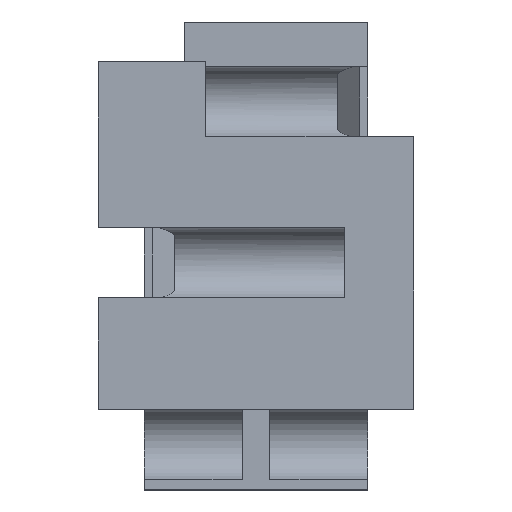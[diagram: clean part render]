
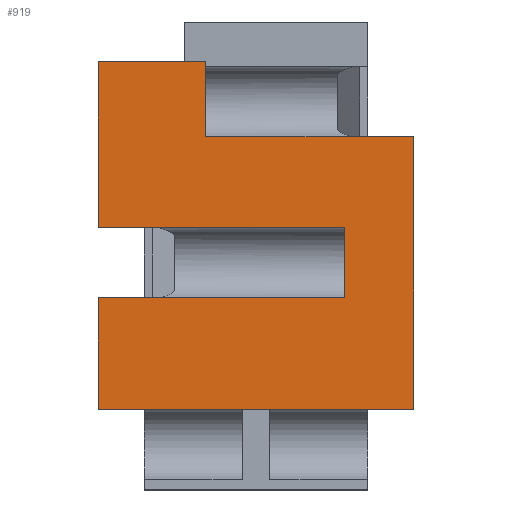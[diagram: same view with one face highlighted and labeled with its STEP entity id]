
A CAD part, top view. The second image highlights one B-rep face of the part: STEP entity #919.
In plain terms, the highlighted planar face has unit normal (0, 0, 1).
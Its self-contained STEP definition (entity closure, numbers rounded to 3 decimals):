
#56=FACE_OUTER_BOUND('',#102,.T.);
#102=EDGE_LOOP('',(#657,#658,#659,#660,#661,#662,#663,#664,#665,#666));
#169=LINE('',#1359,#286);
#174=LINE('',#1369,#291);
#177=LINE('',#1375,#294);
#181=LINE('',#1383,#298);
#183=LINE('',#1387,#300);
#184=LINE('',#1389,#301);
#185=LINE('',#1390,#302);
#186=LINE('',#1391,#303);
#187=LINE('',#1393,#304);
#188=LINE('',#1394,#305);
#286=VECTOR('',#1093,10.);
#291=VECTOR('',#1100,10.);
#294=VECTOR('',#1105,10.);
#298=VECTOR('',#1111,10.);
#300=VECTOR('',#1115,10.);
#301=VECTOR('',#1116,10.);
#302=VECTOR('',#1117,10.);
#303=VECTOR('',#1118,10.);
#304=VECTOR('',#1119,10.);
#305=VECTOR('',#1120,10.);
#400=VERTEX_POINT('',#1356);
#401=VERTEX_POINT('',#1358);
#404=VERTEX_POINT('',#1366);
#405=VERTEX_POINT('',#1368);
#406=VERTEX_POINT('',#1372);
#407=VERTEX_POINT('',#1374);
#410=VERTEX_POINT('',#1382);
#411=VERTEX_POINT('',#1386);
#412=VERTEX_POINT('',#1388);
#413=VERTEX_POINT('',#1392);
#495=EDGE_CURVE('',#401,#400,#169,.T.);
#500=EDGE_CURVE('',#405,#404,#174,.T.);
#503=EDGE_CURVE('',#407,#406,#177,.T.);
#507=EDGE_CURVE('',#410,#407,#181,.T.);
#509=EDGE_CURVE('',#406,#411,#183,.T.);
#510=EDGE_CURVE('',#411,#412,#184,.T.);
#511=EDGE_CURVE('',#412,#405,#185,.T.);
#512=EDGE_CURVE('',#404,#401,#186,.T.);
#513=EDGE_CURVE('',#400,#413,#187,.T.);
#514=EDGE_CURVE('',#413,#410,#188,.T.);
#657=ORIENTED_EDGE('',*,*,#507,.T.);
#658=ORIENTED_EDGE('',*,*,#503,.T.);
#659=ORIENTED_EDGE('',*,*,#509,.T.);
#660=ORIENTED_EDGE('',*,*,#510,.T.);
#661=ORIENTED_EDGE('',*,*,#511,.T.);
#662=ORIENTED_EDGE('',*,*,#500,.T.);
#663=ORIENTED_EDGE('',*,*,#512,.T.);
#664=ORIENTED_EDGE('',*,*,#495,.T.);
#665=ORIENTED_EDGE('',*,*,#513,.T.);
#666=ORIENTED_EDGE('',*,*,#514,.T.);
#876=PLANE('',#982);
#919=ADVANCED_FACE('',(#56),#876,.T.);
#982=AXIS2_PLACEMENT_3D('',#1385,#1113,#1114);
#1093=DIRECTION('',(0.,1.,0.));
#1100=DIRECTION('',(0.,-1.,0.));
#1105=DIRECTION('',(0.,-1.,0.));
#1111=DIRECTION('',(-1.,0.,0.));
#1113=DIRECTION('center_axis',(0.,0.,1.));
#1114=DIRECTION('ref_axis',(1.,0.,0.));
#1115=DIRECTION('',(1.,0.,0.));
#1116=DIRECTION('',(0.,-1.,0.));
#1117=DIRECTION('',(-1.,0.,0.));
#1118=DIRECTION('',(1.,0.,0.));
#1119=DIRECTION('',(-1.,0.,0.));
#1120=DIRECTION('',(0.,1.,0.));
#1356=CARTESIAN_POINT('',(10.3,9.072,11.));
#1358=CARTESIAN_POINT('',(10.3,-8.72,11.));
#1359=CARTESIAN_POINT('',(10.3,9.072,11.));
#1366=CARTESIAN_POINT('',(-10.3,-8.72,11.));
#1368=CARTESIAN_POINT('',(-10.3,-1.458,11.));
#1369=CARTESIAN_POINT('',(-10.3,-1.458,11.));
#1372=CARTESIAN_POINT('',(-10.3,3.142,11.));
#1374=CARTESIAN_POINT('',(-10.3,13.995,11.));
#1375=CARTESIAN_POINT('',(-10.3,3.142,11.));
#1382=CARTESIAN_POINT('',(-3.3,13.995,11.));
#1383=CARTESIAN_POINT('',(-7.3,13.995,11.));
#1385=CARTESIAN_POINT('Origin',(0.,2.638,
11.));
#1386=CARTESIAN_POINT('',(5.8,3.142,11.));
#1387=CARTESIAN_POINT('',(-10.3,3.142,11.));
#1388=CARTESIAN_POINT('',(5.8,-1.458,11.));
#1389=CARTESIAN_POINT('',(5.8,3.142,11.));
#1390=CARTESIAN_POINT('',(-7.3,-1.458,11.));
#1391=CARTESIAN_POINT('',(-7.3,-8.72,11.));
#1392=CARTESIAN_POINT('',(-3.3,9.072,11.));
#1393=CARTESIAN_POINT('',(7.3,9.072,11.));
#1394=CARTESIAN_POINT('',(-3.3,13.995,11.));
